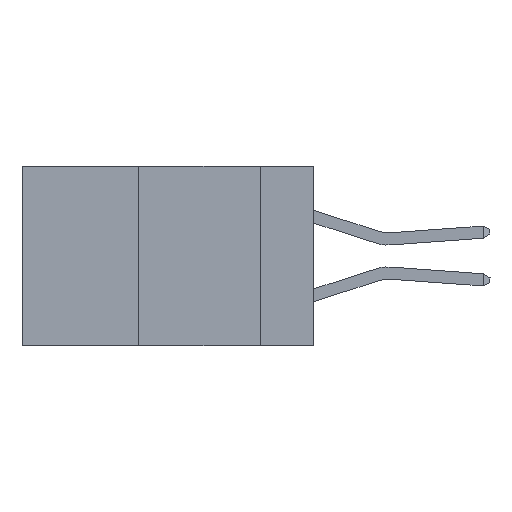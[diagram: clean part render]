
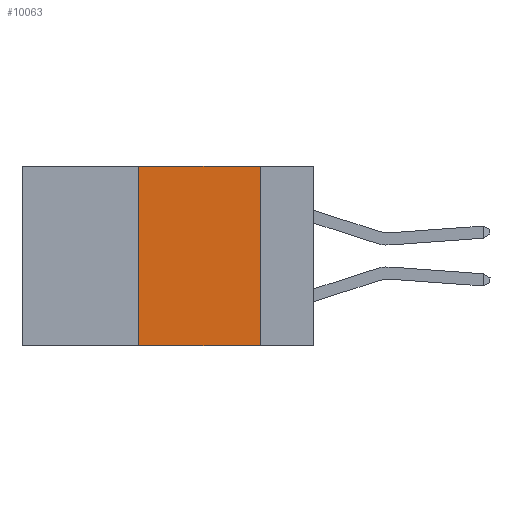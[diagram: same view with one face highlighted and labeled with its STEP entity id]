
A CAD part, left-side view. The second image highlights one B-rep face of the part: STEP entity #10063.
In plain terms, the highlighted planar face has unit normal (-1, 0, 0).
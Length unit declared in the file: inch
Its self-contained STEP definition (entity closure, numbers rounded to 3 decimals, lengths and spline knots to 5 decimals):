
#851 = VERTEX_POINT ( 'NONE', #6392 ) ;
#1923 = CARTESIAN_POINT ( 'NONE',  ( 0., 0.36, 0. ) ) ;
#4661 = DIRECTION ( 'NONE',  ( 0., 0., 1. ) ) ;
#4948 = ORIENTED_EDGE ( 'NONE', *, *, #34801, .F. ) ;
#6030 = CARTESIAN_POINT ( 'NONE',  ( 0., 0.6, 0. ) ) ;
#6386 = DIRECTION ( 'NONE',  ( 1., 0., 0. ) ) ;
#6392 = CARTESIAN_POINT ( 'NONE',  ( 0., 0.11, 0. ) ) ;
#9754 = VERTEX_POINT ( 'NONE', #36932 ) ;
#10063 = ADVANCED_FACE ( 'NONE', ( #34849 ), #25446, .F. ) ;
#11374 = EDGE_CURVE ( 'NONE', #9754, #851, #13991, .T. ) ;
#13826 = VECTOR ( 'NONE', #4661, 39.37008 ) ;
#13991 = LINE ( 'NONE', #6030, #31806 ) ;
#14213 = CARTESIAN_POINT ( 'NONE',  ( 0., 0.6, -0.37 ) ) ;
#14265 = DIRECTION ( 'NONE',  ( 0., 0., -1. ) ) ;
#14538 = AXIS2_PLACEMENT_3D ( 'NONE', #15815, #6386, #22291 ) ;
#14786 = CARTESIAN_POINT ( 'NONE',  ( 0., 0.36, -0.37 ) ) ;
#15064 = EDGE_LOOP ( 'NONE', ( #4948, #35736, #24056, #25006 ) ) ;
#15603 = EDGE_CURVE ( 'NONE', #35459, #33263, #40330, .T. ) ;
#15815 = CARTESIAN_POINT ( 'NONE',  ( 0., 0.6, 0. ) ) ;
#22291 = DIRECTION ( 'NONE',  ( 0., 0., -1. ) ) ;
#23603 = DIRECTION ( 'NONE',  ( 0., -1., 0. ) ) ;
#24056 = ORIENTED_EDGE ( 'NONE', *, *, #37393, .F. ) ;
#25006 = ORIENTED_EDGE ( 'NONE', *, *, #15603, .T. ) ;
#25225 = VECTOR ( 'NONE', #14265, 39.37008 ) ;
#25446 = PLANE ( 'NONE',  #14538 ) ;
#30167 = CARTESIAN_POINT ( 'NONE',  ( 0., 0.11, 0. ) ) ;
#31188 = LINE ( 'NONE', #30167, #25225 ) ;
#31806 = VECTOR ( 'NONE', #35005, 39.37008 ) ;
#33263 = VERTEX_POINT ( 'NONE', #37998 ) ;
#34801 = EDGE_CURVE ( 'NONE', #851, #33263, #31188, .T. ) ;
#34849 = FACE_OUTER_BOUND ( 'NONE', #15064, .T. ) ;
#35005 = DIRECTION ( 'NONE',  ( 0., -1., 0. ) ) ;
#35459 = VERTEX_POINT ( 'NONE', #14786 ) ;
#35736 = ORIENTED_EDGE ( 'NONE', *, *, #11374, .F. ) ;
#36932 = CARTESIAN_POINT ( 'NONE',  ( 0., 0.36, 0. ) ) ;
#37350 = VECTOR ( 'NONE', #23603, 39.37008 ) ;
#37393 = EDGE_CURVE ( 'NONE', #35459, #9754, #40030, .T. ) ;
#37998 = CARTESIAN_POINT ( 'NONE',  ( 0., 0.11, -0.37 ) ) ;
#40030 = LINE ( 'NONE', #1923, #13826 ) ;
#40330 = LINE ( 'NONE', #14213, #37350 ) ;
